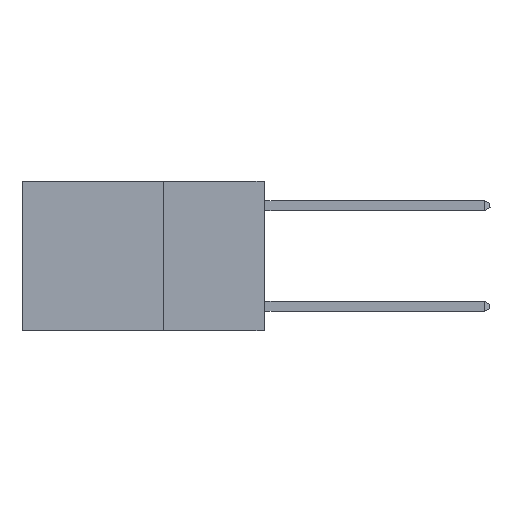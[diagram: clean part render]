
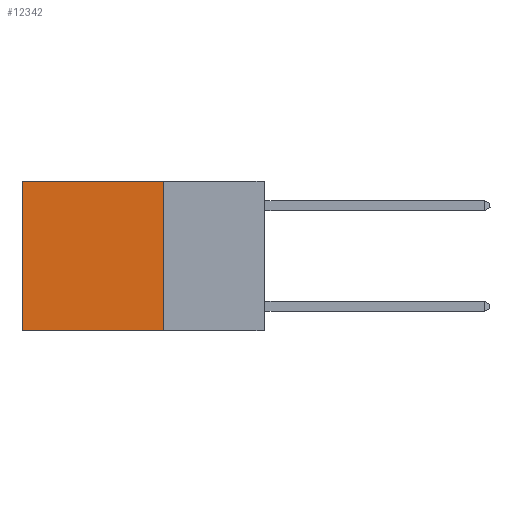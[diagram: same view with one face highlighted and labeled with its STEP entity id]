
A CAD part, left-side view. The second image highlights one B-rep face of the part: STEP entity #12342.
In plain terms, the highlighted planar face has unit normal (-1, 0, 0).
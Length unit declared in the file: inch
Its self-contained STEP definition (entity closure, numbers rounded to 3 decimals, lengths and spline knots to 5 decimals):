
#160 = PLANE ( 'NONE',  #14260 ) ;
#275 = DIRECTION ( 'NONE',  ( 0., 1., 0. ) ) ;
#475 = CARTESIAN_POINT ( 'NONE',  ( 0.2625, 0.25, 0. ) ) ;
#1510 = CARTESIAN_POINT ( 'NONE',  ( 0.2625, 0.25, 0. ) ) ;
#1690 = EDGE_LOOP ( 'NONE', ( #16551, #8136, #9470, #14710 ) ) ;
#2274 = VECTOR ( 'NONE', #4877, 39.37008 ) ;
#2881 = DIRECTION ( 'NONE',  ( 0., 0., -1. ) ) ;
#3494 = CARTESIAN_POINT ( 'NONE',  ( 0.2625, 0.25, -0.37 ) ) ;
#4487 = CARTESIAN_POINT ( 'NONE',  ( 0.2625, 0.25, -0.37 ) ) ;
#4877 = DIRECTION ( 'NONE',  ( 0., 1., 0. ) ) ;
#5942 = DIRECTION ( 'NONE',  ( 0., 0., -1. ) ) ;
#6172 = VERTEX_POINT ( 'NONE', #9914 ) ;
#6655 = EDGE_CURVE ( 'NONE', #6172, #12415, #12340, .T. ) ;
#7273 = CARTESIAN_POINT ( 'NONE',  ( 0.2625, 0.6, -0.37 ) ) ;
#7364 = VERTEX_POINT ( 'NONE', #4487 ) ;
#7778 = FACE_OUTER_BOUND ( 'NONE', #1690, .T. ) ;
#7977 = DIRECTION ( 'NONE',  ( 0., 0., -1. ) ) ;
#8011 = EDGE_CURVE ( 'NONE', #6172, #7364, #11719, .T. ) ;
#8136 = ORIENTED_EDGE ( 'NONE', *, *, #15604, .F. ) ;
#8144 = VECTOR ( 'NONE', #7977, 39.37008 ) ;
#8207 = EDGE_CURVE ( 'NONE', #12415, #10288, #14855, .T. ) ;
#8347 = VECTOR ( 'NONE', #5942, 39.37008 ) ;
#9470 = ORIENTED_EDGE ( 'NONE', *, *, #8011, .F. ) ;
#9914 = CARTESIAN_POINT ( 'NONE',  ( 0.2625, 0.25, 0. ) ) ;
#10288 = VERTEX_POINT ( 'NONE', #7273 ) ;
#10687 = DIRECTION ( 'NONE',  ( 1., 0., 0. ) ) ;
#11719 = LINE ( 'NONE', #475, #8347 ) ;
#11954 = VECTOR ( 'NONE', #275, 39.37008 ) ;
#12340 = LINE ( 'NONE', #13259, #11954 ) ;
#12342 = ADVANCED_FACE ( 'NONE', ( #7778 ), #160, .F. ) ;
#12415 = VERTEX_POINT ( 'NONE', #15821 ) ;
#12614 = LINE ( 'NONE', #3494, #2274 ) ;
#13007 = CARTESIAN_POINT ( 'NONE',  ( 0.2625, 0.6, 0. ) ) ;
#13259 = CARTESIAN_POINT ( 'NONE',  ( 0.2625, 0.25, 0. ) ) ;
#14260 = AXIS2_PLACEMENT_3D ( 'NONE', #1510, #10687, #2881 ) ;
#14710 = ORIENTED_EDGE ( 'NONE', *, *, #6655, .T. ) ;
#14855 = LINE ( 'NONE', #13007, #8144 ) ;
#15604 = EDGE_CURVE ( 'NONE', #7364, #10288, #12614, .T. ) ;
#15821 = CARTESIAN_POINT ( 'NONE',  ( 0.2625, 0.6, 0. ) ) ;
#16551 = ORIENTED_EDGE ( 'NONE', *, *, #8207, .T. ) ;
